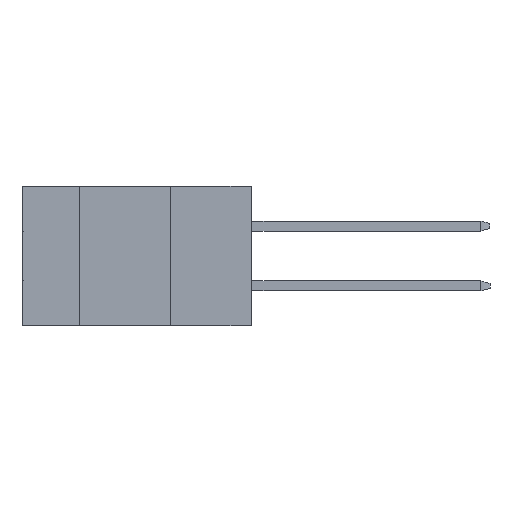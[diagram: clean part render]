
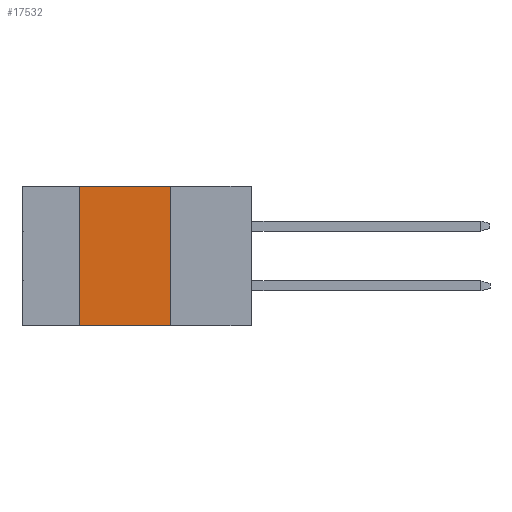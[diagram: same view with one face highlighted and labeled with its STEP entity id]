
A CAD part, left-side view. The second image highlights one B-rep face of the part: STEP entity #17532.
In plain terms, the highlighted planar face has unit normal (-1, 0, 0).
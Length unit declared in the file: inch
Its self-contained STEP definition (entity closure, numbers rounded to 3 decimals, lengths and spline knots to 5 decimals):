
#938 = ORIENTED_EDGE ( 'NONE', *, *, #14388, .T. ) ;
#1273 = CARTESIAN_POINT ( 'NONE',  ( 0., 0.54, 0. ) ) ;
#1500 = DIRECTION ( 'NONE',  ( 0., -1., 0. ) ) ;
#2136 = CARTESIAN_POINT ( 'NONE',  ( 0., 0.254, -0.437 ) ) ;
#3186 = CARTESIAN_POINT ( 'NONE',  ( 0., 0.254, -0.437 ) ) ;
#4366 = CARTESIAN_POINT ( 'NONE',  ( 0., 0.72, 0. ) ) ;
#5040 = EDGE_CURVE ( 'NONE', #7581, #14681, #8210, .T. ) ;
#5703 = EDGE_CURVE ( 'NONE', #14681, #10300, #17466, .T. ) ;
#6447 = VERTEX_POINT ( 'NONE', #19126 ) ;
#6540 = CARTESIAN_POINT ( 'NONE',  ( 0., 0.72, 0. ) ) ;
#7581 = VERTEX_POINT ( 'NONE', #1273 ) ;
#7780 = VECTOR ( 'NONE', #1500, 39.37008 ) ;
#8210 = LINE ( 'NONE', #6540, #7780 ) ;
#9403 = DIRECTION ( 'NONE',  ( 1., 0., 0. ) ) ;
#10300 = VERTEX_POINT ( 'NONE', #3186 ) ;
#10307 = LINE ( 'NONE', #17042, #12648 ) ;
#11359 = ORIENTED_EDGE ( 'NONE', *, *, #21156, .F. ) ;
#12284 = CARTESIAN_POINT ( 'NONE',  ( 0., 0.254, 0. ) ) ;
#12648 = VECTOR ( 'NONE', #13664, 39.37008 ) ;
#13046 = LINE ( 'NONE', #19884, #19597 ) ;
#13057 = ORIENTED_EDGE ( 'NONE', *, *, #5703, .F. ) ;
#13075 = VECTOR ( 'NONE', #20823, 39.37008 ) ;
#13664 = DIRECTION ( 'NONE',  ( 0., -1., 0. ) ) ;
#14388 = EDGE_CURVE ( 'NONE', #6447, #10300, #10307, .T. ) ;
#14434 = FACE_OUTER_BOUND ( 'NONE', #16448, .T. ) ;
#14681 = VERTEX_POINT ( 'NONE', #12284 ) ;
#15986 = AXIS2_PLACEMENT_3D ( 'NONE', #4366, #9403, #21266 ) ;
#16448 = EDGE_LOOP ( 'NONE', ( #13057, #22099, #11359, #938 ) ) ;
#17042 = CARTESIAN_POINT ( 'NONE',  ( 0., 0.72, -0.437 ) ) ;
#17466 = LINE ( 'NONE', #2136, #13075 ) ;
#17532 = ADVANCED_FACE ( 'NONE', ( #14434 ), #19704, .F. ) ;
#19126 = CARTESIAN_POINT ( 'NONE',  ( 0., 0.54, -0.437 ) ) ;
#19548 = DIRECTION ( 'NONE',  ( 0., 0., 1. ) ) ;
#19597 = VECTOR ( 'NONE', #19548, 39.37008 ) ;
#19704 = PLANE ( 'NONE',  #15986 ) ;
#19884 = CARTESIAN_POINT ( 'NONE',  ( 0., 0.54, -0.437 ) ) ;
#20823 = DIRECTION ( 'NONE',  ( 0., 0., -1. ) ) ;
#21156 = EDGE_CURVE ( 'NONE', #6447, #7581, #13046, .T. ) ;
#21266 = DIRECTION ( 'NONE',  ( 0., 0., -1. ) ) ;
#22099 = ORIENTED_EDGE ( 'NONE', *, *, #5040, .F. ) ;
